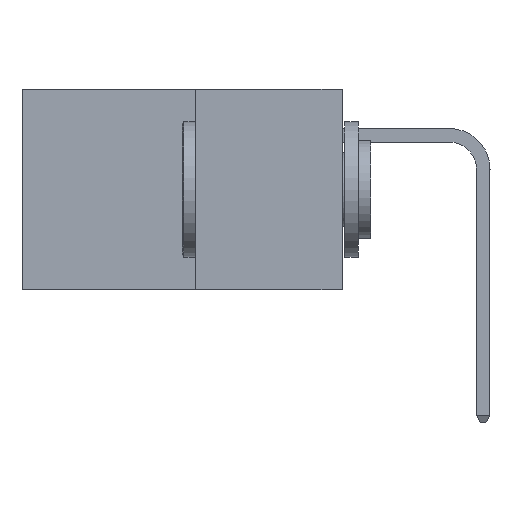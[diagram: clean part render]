
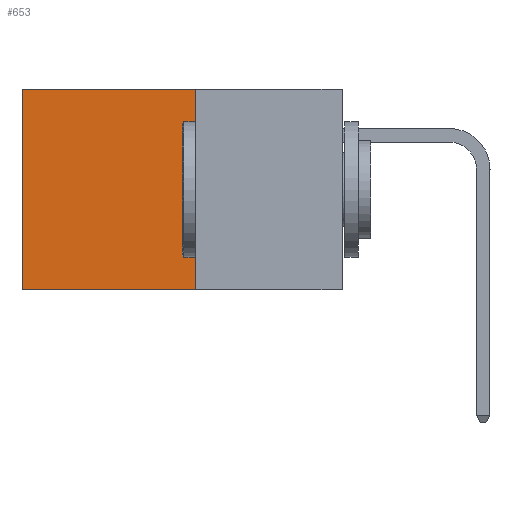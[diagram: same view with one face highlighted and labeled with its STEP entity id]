
A CAD part, left-side view. The second image highlights one B-rep face of the part: STEP entity #653.
In plain terms, the highlighted planar face has unit normal (-1, 0, 0).
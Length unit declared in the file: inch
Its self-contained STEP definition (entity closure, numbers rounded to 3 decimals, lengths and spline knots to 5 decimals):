
#479 = CARTESIAN_POINT ( 'NONE',  ( 0.277, 0.59, -0.37 ) ) ;
#596 = EDGE_CURVE ( 'NONE', #2602, #9206, #6812, .T. ) ;
#653 = ADVANCED_FACE ( 'NONE', ( #5294 ), #2764, .F. ) ;
#705 = VECTOR ( 'NONE', #3490, 39.37008 ) ;
#965 = VERTEX_POINT ( 'NONE', #9774 ) ;
#1247 = ORIENTED_EDGE ( 'NONE', *, *, #4933, .F. ) ;
#1282 = DIRECTION ( 'NONE',  ( 0., 0., -1. ) ) ;
#1296 = CARTESIAN_POINT ( 'NONE',  ( 0.277, 0.27, -0.37 ) ) ;
#1342 = AXIS2_PLACEMENT_3D ( 'NONE', #1296, #2340, #1282 ) ;
#2200 = CARTESIAN_POINT ( 'NONE',  ( 0.277, 0.27, 0. ) ) ;
#2293 = CARTESIAN_POINT ( 'NONE',  ( 0.277, 0.59, 0. ) ) ;
#2340 = DIRECTION ( 'NONE',  ( 1., 0., 0. ) ) ;
#2394 = EDGE_LOOP ( 'NONE', ( #3974, #1247, #6728, #2659 ) ) ;
#2602 = VERTEX_POINT ( 'NONE', #2293 ) ;
#2659 = ORIENTED_EDGE ( 'NONE', *, *, #3498, .T. ) ;
#2764 = PLANE ( 'NONE',  #1342 ) ;
#3060 = DIRECTION ( 'NONE',  ( 0., 1., 0. ) ) ;
#3115 = VECTOR ( 'NONE', #8346, 39.37008 ) ;
#3490 = DIRECTION ( 'NONE',  ( 0., 0., -1. ) ) ;
#3498 = EDGE_CURVE ( 'NONE', #8482, #2602, #7307, .T. ) ;
#3974 = ORIENTED_EDGE ( 'NONE', *, *, #596, .T. ) ;
#4472 = DIRECTION ( 'NONE',  ( 0., 1., 0. ) ) ;
#4675 = CARTESIAN_POINT ( 'NONE',  ( 0.277, 0.27, -0.37 ) ) ;
#4933 = EDGE_CURVE ( 'NONE', #965, #9206, #6955, .T. ) ;
#5116 = VECTOR ( 'NONE', #3060, 39.37008 ) ;
#5294 = FACE_OUTER_BOUND ( 'NONE', #2394, .T. ) ;
#6391 = CARTESIAN_POINT ( 'NONE',  ( 0.277, 0.59, -0.37 ) ) ;
#6728 = ORIENTED_EDGE ( 'NONE', *, *, #8005, .F. ) ;
#6812 = LINE ( 'NONE', #6391, #705 ) ;
#6955 = LINE ( 'NONE', #4675, #8567 ) ;
#7307 = LINE ( 'NONE', #2200, #5116 ) ;
#7640 = CARTESIAN_POINT ( 'NONE',  ( 0.277, 0.27, -0.37 ) ) ;
#8005 = EDGE_CURVE ( 'NONE', #8482, #965, #8982, .T. ) ;
#8346 = DIRECTION ( 'NONE',  ( 0., 0., -1. ) ) ;
#8482 = VERTEX_POINT ( 'NONE', #9315 ) ;
#8567 = VECTOR ( 'NONE', #4472, 39.37008 ) ;
#8982 = LINE ( 'NONE', #7640, #3115 ) ;
#9206 = VERTEX_POINT ( 'NONE', #479 ) ;
#9315 = CARTESIAN_POINT ( 'NONE',  ( 0.277, 0.27, 0. ) ) ;
#9774 = CARTESIAN_POINT ( 'NONE',  ( 0.277, 0.27, -0.37 ) ) ;
